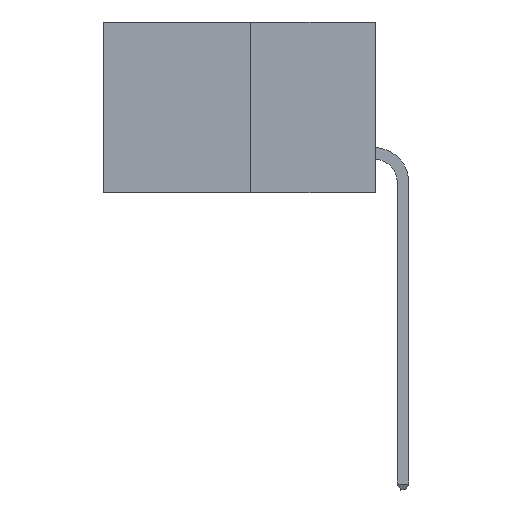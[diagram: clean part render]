
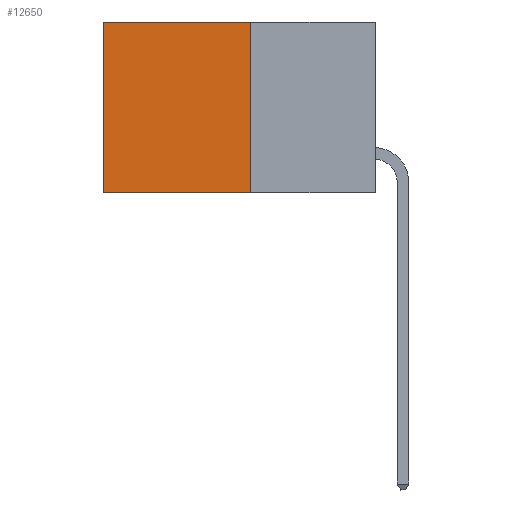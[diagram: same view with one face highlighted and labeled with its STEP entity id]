
A CAD part, left-side view. The second image highlights one B-rep face of the part: STEP entity #12650.
In plain terms, the highlighted planar face has unit normal (-1, 0, 0).
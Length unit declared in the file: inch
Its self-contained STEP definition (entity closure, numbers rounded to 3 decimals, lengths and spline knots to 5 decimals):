
#469 = CARTESIAN_POINT ( 'NONE',  ( 0.277, 0.59, 0. ) ) ;
#658 = EDGE_CURVE ( 'NONE', #4774, #11595, #12053, .T. ) ;
#1908 = DIRECTION ( 'NONE',  ( 0., 1., 0. ) ) ;
#2245 = CARTESIAN_POINT ( 'NONE',  ( 0.277, 0.27, 0. ) ) ;
#2352 = EDGE_CURVE ( 'NONE', #12697, #8244, #7546, .T. ) ;
#2977 = EDGE_CURVE ( 'NONE', #12697, #4774, #3576, .T. ) ;
#3171 = VECTOR ( 'NONE', #6873, 39.37008 ) ;
#3576 = LINE ( 'NONE', #3797, #3171 ) ;
#3797 = CARTESIAN_POINT ( 'NONE',  ( 0.277, 0.27, -0.37 ) ) ;
#4589 = VECTOR ( 'NONE', #1908, 39.37008 ) ;
#4750 = PLANE ( 'NONE',  #13422 ) ;
#4774 = VERTEX_POINT ( 'NONE', #5985 ) ;
#4886 = VECTOR ( 'NONE', #8401, 39.37008 ) ;
#5746 = ORIENTED_EDGE ( 'NONE', *, *, #2352, .T. ) ;
#5905 = DIRECTION ( 'NONE',  ( 1., 0., 0. ) ) ;
#5985 = CARTESIAN_POINT ( 'NONE',  ( 0.277, 0.27, -0.37 ) ) ;
#6158 = ORIENTED_EDGE ( 'NONE', *, *, #2977, .F. ) ;
#6438 = EDGE_CURVE ( 'NONE', #8244, #11595, #7777, .T. ) ;
#6873 = DIRECTION ( 'NONE',  ( 0., 0., -1. ) ) ;
#7546 = LINE ( 'NONE', #8868, #4589 ) ;
#7777 = LINE ( 'NONE', #10393, #4886 ) ;
#8244 = VERTEX_POINT ( 'NONE', #469 ) ;
#8248 = ORIENTED_EDGE ( 'NONE', *, *, #6438, .T. ) ;
#8401 = DIRECTION ( 'NONE',  ( 0., 0., -1. ) ) ;
#8868 = CARTESIAN_POINT ( 'NONE',  ( 0.277, 0.27, 0. ) ) ;
#9025 = CARTESIAN_POINT ( 'NONE',  ( 0.277, 0.59, -0.37 ) ) ;
#10096 = CARTESIAN_POINT ( 'NONE',  ( 0.277, 0.27, -0.37 ) ) ;
#10393 = CARTESIAN_POINT ( 'NONE',  ( 0.277, 0.59, -0.37 ) ) ;
#11508 = DIRECTION ( 'NONE',  ( 0., 1., 0. ) ) ;
#11595 = VERTEX_POINT ( 'NONE', #9025 ) ;
#12053 = LINE ( 'NONE', #14435, #14433 ) ;
#12365 = ORIENTED_EDGE ( 'NONE', *, *, #658, .F. ) ;
#12583 = FACE_OUTER_BOUND ( 'NONE', #13882, .T. ) ;
#12650 = ADVANCED_FACE ( 'NONE', ( #12583 ), #4750, .F. ) ;
#12697 = VERTEX_POINT ( 'NONE', #2245 ) ;
#13225 = DIRECTION ( 'NONE',  ( 0., 0., -1. ) ) ;
#13422 = AXIS2_PLACEMENT_3D ( 'NONE', #10096, #5905, #13225 ) ;
#13882 = EDGE_LOOP ( 'NONE', ( #8248, #12365, #6158, #5746 ) ) ;
#14433 = VECTOR ( 'NONE', #11508, 39.37008 ) ;
#14435 = CARTESIAN_POINT ( 'NONE',  ( 0.277, 0.27, -0.37 ) ) ;
